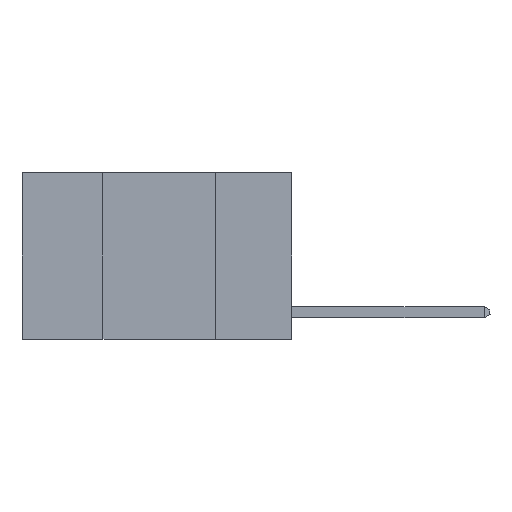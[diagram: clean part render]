
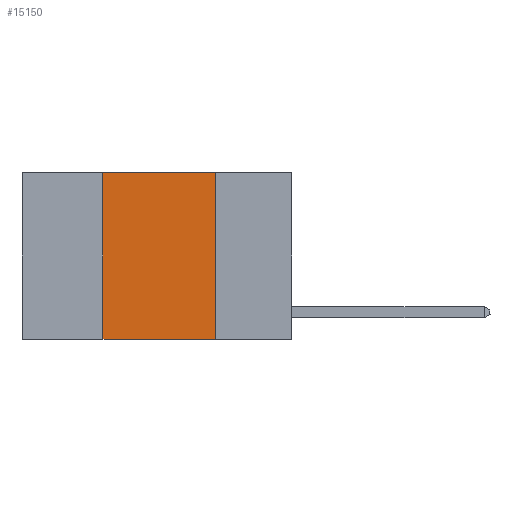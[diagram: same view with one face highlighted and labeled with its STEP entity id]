
A CAD part, left-side view. The second image highlights one B-rep face of the part: STEP entity #15150.
In plain terms, the highlighted planar face has unit normal (-1, 0, 0).
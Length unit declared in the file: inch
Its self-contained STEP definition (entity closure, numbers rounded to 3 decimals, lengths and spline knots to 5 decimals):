
#201 = EDGE_CURVE ( 'NONE', #5088, #21987, #9756, .T. ) ;
#316 = VECTOR ( 'NONE', #17087, 39.37008 ) ;
#890 = DIRECTION ( 'NONE',  ( 1., 0., 0. ) ) ;
#1026 = ORIENTED_EDGE ( 'NONE', *, *, #6832, .F. ) ;
#1896 = EDGE_LOOP ( 'NONE', ( #2965, #1026, #21895, #4732 ) ) ;
#2432 = LINE ( 'NONE', #11188, #10778 ) ;
#2965 = ORIENTED_EDGE ( 'NONE', *, *, #7572, .F. ) ;
#4732 = ORIENTED_EDGE ( 'NONE', *, *, #201, .T. ) ;
#4814 = DIRECTION ( 'NONE',  ( 0., 0., 1. ) ) ;
#5054 = CARTESIAN_POINT ( 'NONE',  ( 0., 0.42, 0. ) ) ;
#5088 = VERTEX_POINT ( 'NONE', #10511 ) ;
#6070 = DIRECTION ( 'NONE',  ( 0., 0., -1. ) ) ;
#6118 = EDGE_CURVE ( 'NONE', #5088, #8624, #18606, .T. ) ;
#6170 = DIRECTION ( 'NONE',  ( 0., -1., 0. ) ) ;
#6832 = EDGE_CURVE ( 'NONE', #8624, #15294, #9700, .T. ) ;
#7424 = AXIS2_PLACEMENT_3D ( 'NONE', #12269, #890, #6070 ) ;
#7572 = EDGE_CURVE ( 'NONE', #15294, #21987, #2432, .T. ) ;
#8609 = CARTESIAN_POINT ( 'NONE',  ( 0., 0.42, 0. ) ) ;
#8624 = VERTEX_POINT ( 'NONE', #8609 ) ;
#9287 = VECTOR ( 'NONE', #6170, 39.37008 ) ;
#9396 = DIRECTION ( 'NONE',  ( 0., 0., -1. ) ) ;
#9700 = LINE ( 'NONE', #16622, #316 ) ;
#9756 = LINE ( 'NONE', #19940, #9287 ) ;
#9863 = CARTESIAN_POINT ( 'NONE',  ( 0., 0.17, -0.37 ) ) ;
#10495 = PLANE ( 'NONE',  #7424 ) ;
#10511 = CARTESIAN_POINT ( 'NONE',  ( 0., 0.42, -0.37 ) ) ;
#10778 = VECTOR ( 'NONE', #9396, 39.37008 ) ;
#11188 = CARTESIAN_POINT ( 'NONE',  ( 0., 0.17, 0. ) ) ;
#11220 = FACE_OUTER_BOUND ( 'NONE', #1896, .T. ) ;
#12269 = CARTESIAN_POINT ( 'NONE',  ( 0., 0.6, 0. ) ) ;
#14328 = VECTOR ( 'NONE', #4814, 39.37008 ) ;
#15150 = ADVANCED_FACE ( 'NONE', ( #11220 ), #10495, .F. ) ;
#15294 = VERTEX_POINT ( 'NONE', #20280 ) ;
#16622 = CARTESIAN_POINT ( 'NONE',  ( 0., 0.6, 0. ) ) ;
#17087 = DIRECTION ( 'NONE',  ( 0., -1., 0. ) ) ;
#18606 = LINE ( 'NONE', #5054, #14328 ) ;
#19940 = CARTESIAN_POINT ( 'NONE',  ( 0., 0.6, -0.37 ) ) ;
#20280 = CARTESIAN_POINT ( 'NONE',  ( 0., 0.17, 0. ) ) ;
#21895 = ORIENTED_EDGE ( 'NONE', *, *, #6118, .F. ) ;
#21987 = VERTEX_POINT ( 'NONE', #9863 ) ;
